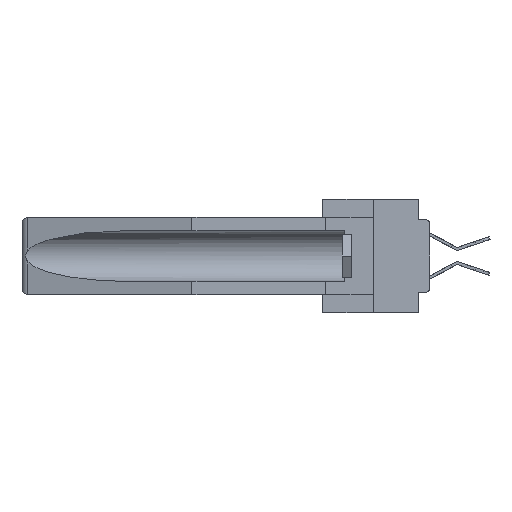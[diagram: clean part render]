
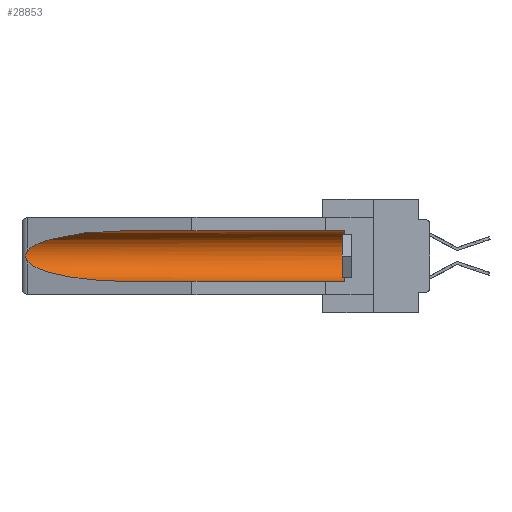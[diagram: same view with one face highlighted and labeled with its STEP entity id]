
A CAD part, left-side view. The second image highlights one B-rep face of the part: STEP entity #28853.
In plain terms, the highlighted cylindrical face has radius 2.857 mm (diameter 5.715 mm), a partial arc.
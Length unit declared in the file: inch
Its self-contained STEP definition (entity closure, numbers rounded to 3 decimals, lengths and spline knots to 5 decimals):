
#833 = CARTESIAN_POINT ( 'NONE',  ( 0.21114, 1.30732, -0.284 ) ) ;
#970 = VERTEX_POINT ( 'NONE', #34887 ) ;
#1124 = VECTOR ( 'NONE', #6835, 39.37008 ) ;
#1931 = EDGE_CURVE ( 'NONE', #6733, #35595, #2882, .T. ) ;
#1932 = VERTEX_POINT ( 'NONE', #14475 ) ;
#2184 = CARTESIAN_POINT ( 'NONE',  ( 0.155, 0.126, -0.059 ) ) ;
#2188 = CARTESIAN_POINT ( 'NONE',  ( 0.26655, 1.53094, -0.18657 ) ) ;
#2882 = LINE ( 'NONE', #22879, #19075 ) ;
#3605 = AXIS2_PLACEMENT_3D ( 'NONE', #10507, #7847, #4858 ) ;
#3896 = EDGE_CURVE ( 'NONE', #35595, #14619, #29407, .T. ) ;
#4858 = DIRECTION ( 'NONE',  ( 0., 0., 1. ) ) ;
#6401 = ORIENTED_EDGE ( 'NONE', *, *, #3896, .T. ) ;
#6733 = VERTEX_POINT ( 'NONE', #2184 ) ;
#6835 = DIRECTION ( 'NONE',  ( 0., 1., 0. ) ) ;
#6930 = LINE ( 'NONE', #26967, #1124 ) ;
#7226 =( BOUNDED_CURVE ( )  B_SPLINE_CURVE ( 3, ( #29864, #9492, #833, #26959 ),
 .UNSPECIFIED., .F., .F. ) 
 B_SPLINE_CURVE_WITH_KNOTS ( ( 4, 4 ),
 ( 0.1948, 1.5708 ),
 .UNSPECIFIED. ) 
 CURVE ( )  GEOMETRIC_REPRESENTATION_ITEM ( )  RATIONAL_B_SPLINE_CURVE ( ( 1., 0.848, 0.848, 1. ) ) 
 REPRESENTATION_ITEM ( '' )  );
#7686 = CARTESIAN_POINT ( 'NONE',  ( 0.2673, 1.5327, -0.16383 ) ) ;
#7804 = CARTESIAN_POINT ( 'NONE',  ( 0.2675, 1.53308, -0.16763 ) ) ;
#7847 = DIRECTION ( 'NONE',  ( 0., -1., 0. ) ) ;
#7933 = CARTESIAN_POINT ( 'NONE',  ( 0.26537, 1.52718, -0.14972 ) ) ;
#8984 = ORIENTED_EDGE ( 'NONE', *, *, #1931, .T. ) ;
#9492 = CARTESIAN_POINT ( 'NONE',  ( 0.25451, 1.48313, -0.24835 ) ) ;
#10467 = CARTESIAN_POINT ( 'NONE',  ( 0.26597, 1.52961, -0.15275 ) ) ;
#10507 = CARTESIAN_POINT ( 'NONE',  ( 0.155, 0.126, -0.1715 ) ) ;
#10656 = CARTESIAN_POINT ( 'NONE',  ( 0.26537, 1.52718, -0.19328 ) ) ;
#12260 = AXIS2_PLACEMENT_3D ( 'NONE', #25566, #20048, #17165 ) ;
#13279 = ORIENTED_EDGE ( 'NONE', *, *, #19166, .T. ) ;
#14475 = CARTESIAN_POINT ( 'NONE',  ( 0.155, 0.126, -0.284 ) ) ;
#14619 = VERTEX_POINT ( 'NONE', #26715 ) ;
#15700 = EDGE_CURVE ( 'NONE', #14619, #32692, #19918, .T. ) ;
#17165 = DIRECTION ( 'NONE',  ( 0., 0., 1. ) ) ;
#18963 = EDGE_CURVE ( 'NONE', #32692, #970, #7226, .T. ) ;
#19075 = VECTOR ( 'NONE', #22996, 39.37008 ) ;
#19166 = EDGE_CURVE ( 'NONE', #1932, #6733, #32906, .T. ) ;
#19377 = CARTESIAN_POINT ( 'NONE',  ( 0.2675, 1.53308, -0.17534 ) ) ;
#19918 = B_SPLINE_CURVE_WITH_KNOTS ( 'NONE', 3,
 ( #33611, #10467, #36663, #7686, #7804, #19377, #33742, #2188, #22279, #25158 ),
 .UNSPECIFIED., .F., .F.,
 ( 4, 2, 2, 2, 4 ),
 ( 0., 0.00029, 0.00058, 0.00087, 0.00117 ),
 .UNSPECIFIED. ) ;
#20048 = DIRECTION ( 'NONE',  ( 0., 1., 0. ) ) ;
#21942 = EDGE_LOOP ( 'NONE', ( #6401, #34247, #22105, #27019, #13279, #8984 ) ) ;
#22105 = ORIENTED_EDGE ( 'NONE', *, *, #18963, .T. ) ;
#22279 = CARTESIAN_POINT ( 'NONE',  ( 0.26597, 1.5296, -0.19026 ) ) ;
#22879 = CARTESIAN_POINT ( 'NONE',  ( 0.155, -0.30754, -0.059 ) ) ;
#22996 = DIRECTION ( 'NONE',  ( 0., 1., 0. ) ) ;
#23877 = EDGE_CURVE ( 'NONE', #1932, #970, #6930, .T. ) ;
#25158 = CARTESIAN_POINT ( 'NONE',  ( 0.26537, 1.52718, -0.19328 ) ) ;
#25566 = CARTESIAN_POINT ( 'NONE',  ( 0.155, -0.30754, -0.1715 ) ) ;
#25929 = CYLINDRICAL_SURFACE ( 'NONE', #12260, 0.1125 ) ;
#26715 = CARTESIAN_POINT ( 'NONE',  ( 0.26537, 1.52718, -0.14972 ) ) ;
#26959 = CARTESIAN_POINT ( 'NONE',  ( 0.155, 1.07973, -0.284 ) ) ;
#26967 = CARTESIAN_POINT ( 'NONE',  ( 0.155, -0.30754, -0.284 ) ) ;
#27019 = ORIENTED_EDGE ( 'NONE', *, *, #23877, .F. ) ;
#28203 = CARTESIAN_POINT ( 'NONE',  ( 0.21114, 1.30732, -0.059 ) ) ;
#28853 = ADVANCED_FACE ( 'NONE', ( #33610 ), #25929, .F. ) ;
#29407 =( BOUNDED_CURVE ( )  B_SPLINE_CURVE ( 3, ( #34263, #28203, #36665, #7933 ),
 .UNSPECIFIED., .F., .F. ) 
 B_SPLINE_CURVE_WITH_KNOTS ( ( 4, 4 ),
 ( 4.71239, 6.08839 ),
 .UNSPECIFIED. ) 
 CURVE ( )  GEOMETRIC_REPRESENTATION_ITEM ( )  RATIONAL_B_SPLINE_CURVE ( ( 1., 0.848, 0.848, 1. ) ) 
 REPRESENTATION_ITEM ( '' )  );
#29864 = CARTESIAN_POINT ( 'NONE',  ( 0.26537, 1.52718, -0.19328 ) ) ;
#32692 = VERTEX_POINT ( 'NONE', #10656 ) ;
#32906 = CIRCLE ( 'NONE', #3605, 0.1125 ) ;
#33610 = FACE_OUTER_BOUND ( 'NONE', #21942, .T. ) ;
#33611 = CARTESIAN_POINT ( 'NONE',  ( 0.26537, 1.52718, -0.14972 ) ) ;
#33742 = CARTESIAN_POINT ( 'NONE',  ( 0.2673, 1.53269, -0.17917 ) ) ;
#33874 = CARTESIAN_POINT ( 'NONE',  ( 0.155, 1.07973, -0.059 ) ) ;
#34247 = ORIENTED_EDGE ( 'NONE', *, *, #15700, .T. ) ;
#34263 = CARTESIAN_POINT ( 'NONE',  ( 0.155, 1.07973, -0.059 ) ) ;
#34887 = CARTESIAN_POINT ( 'NONE',  ( 0.155, 1.07973, -0.284 ) ) ;
#35595 = VERTEX_POINT ( 'NONE', #33874 ) ;
#36663 = CARTESIAN_POINT ( 'NONE',  ( 0.26654, 1.53092, -0.15636 ) ) ;
#36665 = CARTESIAN_POINT ( 'NONE',  ( 0.25451, 1.48313, -0.09465 ) ) ;
